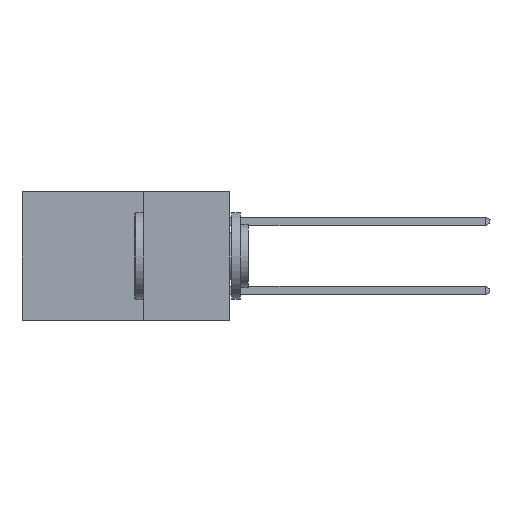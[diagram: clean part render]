
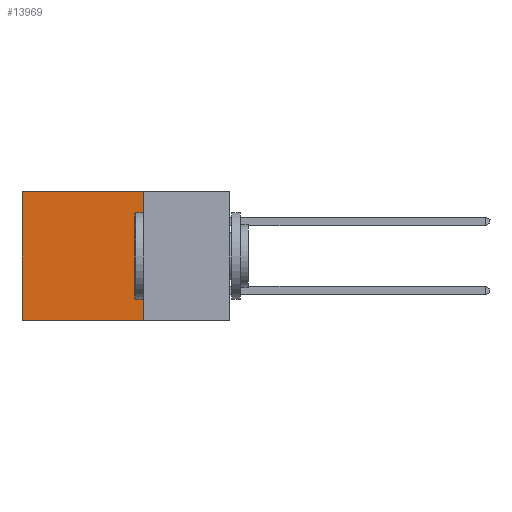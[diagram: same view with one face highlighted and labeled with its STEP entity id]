
A CAD part, left-side view. The second image highlights one B-rep face of the part: STEP entity #13969.
In plain terms, the highlighted planar face has unit normal (-1, 0, 0).
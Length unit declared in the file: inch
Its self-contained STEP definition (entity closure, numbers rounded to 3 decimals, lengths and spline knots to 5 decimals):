
#1559 = VERTEX_POINT ( 'NONE', #26070 ) ;
#1755 = DIRECTION ( 'NONE',  ( 0., 1., 0. ) ) ;
#2639 = VECTOR ( 'NONE', #11613, 39.37008 ) ;
#3188 = LINE ( 'NONE', #9455, #6265 ) ;
#3802 = CARTESIAN_POINT ( 'NONE',  ( 0.2615, 0.25, 0. ) ) ;
#4036 = EDGE_CURVE ( 'NONE', #20457, #1559, #3188, .T. ) ;
#4311 = AXIS2_PLACEMENT_3D ( 'NONE', #26670, #7923, #22690 ) ;
#4349 = CARTESIAN_POINT ( 'NONE',  ( 0.2615, 0.6, 0. ) ) ;
#4738 = VERTEX_POINT ( 'NONE', #4349 ) ;
#5758 = VECTOR ( 'NONE', #1755, 39.37008 ) ;
#6265 = VECTOR ( 'NONE', #25756, 39.37008 ) ;
#6504 = FACE_OUTER_BOUND ( 'NONE', #9839, .T. ) ;
#7146 = EDGE_CURVE ( 'NONE', #4738, #20413, #9535, .T. ) ;
#7923 = DIRECTION ( 'NONE',  ( 1., 0., 0. ) ) ;
#9363 = ORIENTED_EDGE ( 'NONE', *, *, #7146, .T. ) ;
#9455 = CARTESIAN_POINT ( 'NONE',  ( 0.2615, 0.25, -0.37 ) ) ;
#9535 = LINE ( 'NONE', #18142, #16367 ) ;
#9839 = EDGE_LOOP ( 'NONE', ( #9363, #20646, #20478, #24028 ) ) ;
#11613 = DIRECTION ( 'NONE',  ( 0., 1., 0. ) ) ;
#12764 = PLANE ( 'NONE',  #4311 ) ;
#13969 = ADVANCED_FACE ( 'NONE', ( #6504 ), #12764, .F. ) ;
#15854 = CARTESIAN_POINT ( 'NONE',  ( 0.2615, 0.25, -0.37 ) ) ;
#16331 = EDGE_CURVE ( 'NONE', #1559, #20413, #22030, .T. ) ;
#16367 = VECTOR ( 'NONE', #22134, 39.37008 ) ;
#17743 = CARTESIAN_POINT ( 'NONE',  ( 0.2615, 0.6, -0.37 ) ) ;
#17879 = CARTESIAN_POINT ( 'NONE',  ( 0.2615, 0.25, 0. ) ) ;
#18142 = CARTESIAN_POINT ( 'NONE',  ( 0.2615, 0.6, -0.37 ) ) ;
#20413 = VERTEX_POINT ( 'NONE', #17743 ) ;
#20457 = VERTEX_POINT ( 'NONE', #17879 ) ;
#20478 = ORIENTED_EDGE ( 'NONE', *, *, #4036, .F. ) ;
#20646 = ORIENTED_EDGE ( 'NONE', *, *, #16331, .F. ) ;
#22030 = LINE ( 'NONE', #15854, #2639 ) ;
#22044 = EDGE_CURVE ( 'NONE', #20457, #4738, #22531, .T. ) ;
#22134 = DIRECTION ( 'NONE',  ( 0., 0., -1. ) ) ;
#22531 = LINE ( 'NONE', #3802, #5758 ) ;
#22690 = DIRECTION ( 'NONE',  ( 0., 0., -1. ) ) ;
#24028 = ORIENTED_EDGE ( 'NONE', *, *, #22044, .T. ) ;
#25756 = DIRECTION ( 'NONE',  ( 0., 0., -1. ) ) ;
#26070 = CARTESIAN_POINT ( 'NONE',  ( 0.2615, 0.25, -0.37 ) ) ;
#26670 = CARTESIAN_POINT ( 'NONE',  ( 0.2615, 0.25, -0.37 ) ) ;
